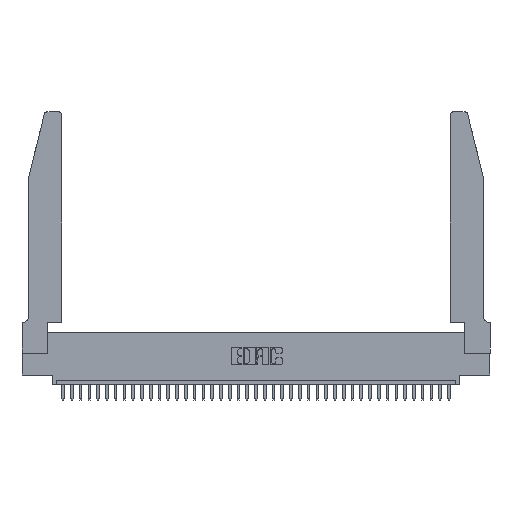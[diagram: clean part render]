
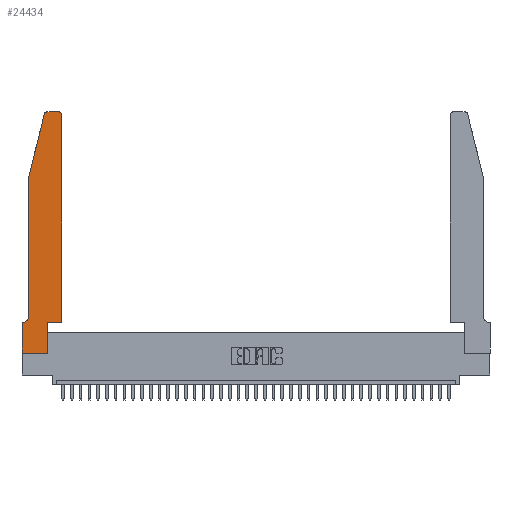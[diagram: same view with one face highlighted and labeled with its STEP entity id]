
A CAD part, top view. The second image highlights one B-rep face of the part: STEP entity #24434.
In plain terms, the highlighted planar face has unit normal (0, 0, 1).
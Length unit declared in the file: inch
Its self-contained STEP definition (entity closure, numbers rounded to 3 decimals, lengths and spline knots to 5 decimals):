
#1061 = CIRCLE ( 'NONE', #25714, 0.07 ) ;
#1182 = VERTEX_POINT ( 'NONE', #9189 ) ;
#1432 = PLANE ( 'NONE',  #14011 ) ;
#1467 = EDGE_CURVE ( 'NONE', #1182, #26099, #12471, .T. ) ;
#1589 = VECTOR ( 'NONE', #28318, 39.37008 ) ;
#2331 = DIRECTION ( 'NONE',  ( 0., 1., 0. ) ) ;
#2900 = ORIENTED_EDGE ( 'NONE', *, *, #17953, .T. ) ;
#3769 = VERTEX_POINT ( 'NONE', #27528 ) ;
#4047 = CARTESIAN_POINT ( 'NONE',  ( 0., 0.35, 0.37 ) ) ;
#4171 = DIRECTION ( 'NONE',  ( 1., 0., 0. ) ) ;
#4356 = DIRECTION ( 'NONE',  ( 0., -1., 0. ) ) ;
#4903 = ORIENTED_EDGE ( 'NONE', *, *, #36880, .T. ) ;
#4927 = CARTESIAN_POINT ( 'NONE',  ( 0.2865, 0., 0.37 ) ) ;
#5087 = DIRECTION ( 'NONE',  ( 1., 0., 0. ) ) ;
#5331 = CARTESIAN_POINT ( 'NONE',  ( 0.4505, 0.35, 0.37 ) ) ;
#5614 = AXIS2_PLACEMENT_3D ( 'NONE', #38301, #8611, #5087 ) ;
#5818 = DIRECTION ( 'NONE',  ( 1., 0., 0. ) ) ;
#6671 = VECTOR ( 'NONE', #12154, 39.37008 ) ;
#6761 = VECTOR ( 'NONE', #11085, 39.37008 ) ;
#6968 = ORIENTED_EDGE ( 'NONE', *, *, #31819, .T. ) ;
#7030 = ORIENTED_EDGE ( 'NONE', *, *, #17607, .T. ) ;
#8611 = DIRECTION ( 'NONE',  ( 0., 0., 1. ) ) ;
#9189 = CARTESIAN_POINT ( 'NONE',  ( 0.4505, 0.35, 0.37 ) ) ;
#9821 = VERTEX_POINT ( 'NONE', #28279 ) ;
#9985 = CARTESIAN_POINT ( 'NONE',  ( 0.284, 2.75, 0.37 ) ) ;
#10207 = CARTESIAN_POINT ( 'NONE',  ( 0., 0., 0.37 ) ) ;
#10769 = VERTEX_POINT ( 'NONE', #4927 ) ;
#10833 = DIRECTION ( 'NONE',  ( 0., 0., 1. ) ) ;
#10974 = LINE ( 'NONE', #11560, #12807 ) ;
#11085 = DIRECTION ( 'NONE',  ( 1., 0., 0. ) ) ;
#11218 = CARTESIAN_POINT ( 'NONE',  ( 0., 0.35, 0.37 ) ) ;
#11560 = CARTESIAN_POINT ( 'NONE',  ( 0., 0., 0.37 ) ) ;
#12154 = DIRECTION ( 'NONE',  ( 0., -1., 0. ) ) ;
#12471 = LINE ( 'NONE', #26044, #14356 ) ;
#12807 = VECTOR ( 'NONE', #5818, 39.37008 ) ;
#12942 = CARTESIAN_POINT ( 'NONE',  ( 0.4505, 2.72, 0.37 ) ) ;
#13210 = VERTEX_POINT ( 'NONE', #36786 ) ;
#13451 = CARTESIAN_POINT ( 'NONE',  ( 0.2605, 2.75, 0.37 ) ) ;
#13801 = LINE ( 'NONE', #14309, #17945 ) ;
#14011 = AXIS2_PLACEMENT_3D ( 'NONE', #4047, #34203, #4171 ) ;
#14309 = CARTESIAN_POINT ( 'NONE',  ( 0.2865, 0.35, 0.37 ) ) ;
#14356 = VECTOR ( 'NONE', #34389, 39.37008 ) ;
#15005 = EDGE_CURVE ( 'NONE', #3769, #16495, #18680, .T. ) ;
#15576 = EDGE_CURVE ( 'NONE', #35064, #13210, #21445, .T. ) ;
#16495 = VERTEX_POINT ( 'NONE', #9985 ) ;
#16555 = DIRECTION ( 'NONE',  ( -1., 0., 0. ) ) ;
#17607 = EDGE_CURVE ( 'NONE', #26099, #3769, #23676, .T. ) ;
#17945 = VECTOR ( 'NONE', #2331, 39.37008 ) ;
#17953 = EDGE_CURVE ( 'NONE', #16495, #23652, #18873, .T. ) ;
#18583 = VERTEX_POINT ( 'NONE', #32148 ) ;
#18680 = LINE ( 'NONE', #13451, #32659 ) ;
#18739 = ORIENTED_EDGE ( 'NONE', *, *, #28332, .T. ) ;
#18873 = CIRCLE ( 'NONE', #33743, 0.03 ) ;
#20123 = CARTESIAN_POINT ( 'NONE',  ( 0.0755, 2., 0.37 ) ) ;
#20349 = DIRECTION ( 'NONE',  ( -1., 0., 0. ) ) ;
#20697 = LINE ( 'NONE', #36657, #1589 ) ;
#21445 = LINE ( 'NONE', #10207, #33500 ) ;
#23557 = LINE ( 'NONE', #26922, #6671 ) ;
#23652 = VERTEX_POINT ( 'NONE', #24561 ) ;
#23676 = CIRCLE ( 'NONE', #5614, 0.03 ) ;
#23727 = CARTESIAN_POINT ( 'NONE',  ( 0.0755, 0.42, 0.37 ) ) ;
#24434 = ADVANCED_FACE ( 'NONE', ( #28922 ), #1432, .T. ) ;
#24514 = EDGE_CURVE ( 'NONE', #9821, #35064, #30726, .T. ) ;
#24561 = CARTESIAN_POINT ( 'NONE',  ( 0.25487, 2.72718, 0.37 ) ) ;
#25319 = CARTESIAN_POINT ( 'NONE',  ( 0.284, 2.72, 0.37 ) ) ;
#25714 = AXIS2_PLACEMENT_3D ( 'NONE', #29087, #26383, #32180 ) ;
#25818 = ORIENTED_EDGE ( 'NONE', *, *, #37059, .T. ) ;
#26044 = CARTESIAN_POINT ( 'NONE',  ( 0.4505, 0.35, 0.37 ) ) ;
#26099 = VERTEX_POINT ( 'NONE', #12942 ) ;
#26196 = VERTEX_POINT ( 'NONE', #20123 ) ;
#26383 = DIRECTION ( 'NONE',  ( 0., 0., -1. ) ) ;
#26922 = CARTESIAN_POINT ( 'NONE',  ( 0.0755, 2., 0.37 ) ) ;
#27528 = CARTESIAN_POINT ( 'NONE',  ( 0.4205, 2.75, 0.37 ) ) ;
#27749 = ORIENTED_EDGE ( 'NONE', *, *, #1467, .T. ) ;
#28279 = CARTESIAN_POINT ( 'NONE',  ( 0.0055, 0.35, 0.37 ) ) ;
#28318 = DIRECTION ( 'NONE',  ( -0.239, -0.971, 0. ) ) ;
#28332 = EDGE_CURVE ( 'NONE', #36192, #9821, #1061, .T. ) ;
#28559 = DIRECTION ( 'NONE',  ( 1., 0., 0. ) ) ;
#28863 = ORIENTED_EDGE ( 'NONE', *, *, #15576, .T. ) ;
#28922 = FACE_OUTER_BOUND ( 'NONE', #34156, .T. ) ;
#29087 = CARTESIAN_POINT ( 'NONE',  ( 0.0055, 0.42, 0.37 ) ) ;
#29350 = ORIENTED_EDGE ( 'NONE', *, *, #31840, .T. ) ;
#29849 = ORIENTED_EDGE ( 'NONE', *, *, #34517, .T. ) ;
#30540 = LINE ( 'NONE', #5331, #6761 ) ;
#30726 = LINE ( 'NONE', #35471, #34892 ) ;
#31819 = EDGE_CURVE ( 'NONE', #10769, #18583, #13801, .T. ) ;
#31840 = EDGE_CURVE ( 'NONE', #18583, #1182, #30540, .T. ) ;
#32148 = CARTESIAN_POINT ( 'NONE',  ( 0.2865, 0.35, 0.37 ) ) ;
#32180 = DIRECTION ( 'NONE',  ( -1., 0., 0. ) ) ;
#32659 = VECTOR ( 'NONE', #20349, 39.37008 ) ;
#33500 = VECTOR ( 'NONE', #4356, 39.37008 ) ;
#33657 = ORIENTED_EDGE ( 'NONE', *, *, #15005, .T. ) ;
#33743 = AXIS2_PLACEMENT_3D ( 'NONE', #25319, #10833, #28559 ) ;
#34156 = EDGE_LOOP ( 'NONE', ( #33657, #2900, #29849, #25818, #18739, #38175, #28863, #4903, #6968, #29350, #27749, #7030 ) ) ;
#34203 = DIRECTION ( 'NONE',  ( 0., 0., 1. ) ) ;
#34389 = DIRECTION ( 'NONE',  ( 0., 1., 0. ) ) ;
#34517 = EDGE_CURVE ( 'NONE', #23652, #26196, #20697, .T. ) ;
#34892 = VECTOR ( 'NONE', #16555, 39.37008 ) ;
#35064 = VERTEX_POINT ( 'NONE', #11218 ) ;
#35471 = CARTESIAN_POINT ( 'NONE',  ( 0.0755, 0.35, 0.37 ) ) ;
#36192 = VERTEX_POINT ( 'NONE', #23727 ) ;
#36657 = CARTESIAN_POINT ( 'NONE',  ( 0.0755, 2., 0.37 ) ) ;
#36786 = CARTESIAN_POINT ( 'NONE',  ( 0., 0., 0.37 ) ) ;
#36880 = EDGE_CURVE ( 'NONE', #13210, #10769, #10974, .T. ) ;
#37059 = EDGE_CURVE ( 'NONE', #26196, #36192, #23557, .T. ) ;
#38175 = ORIENTED_EDGE ( 'NONE', *, *, #24514, .T. ) ;
#38301 = CARTESIAN_POINT ( 'NONE',  ( 0.4205, 2.72, 0.37 ) ) ;
